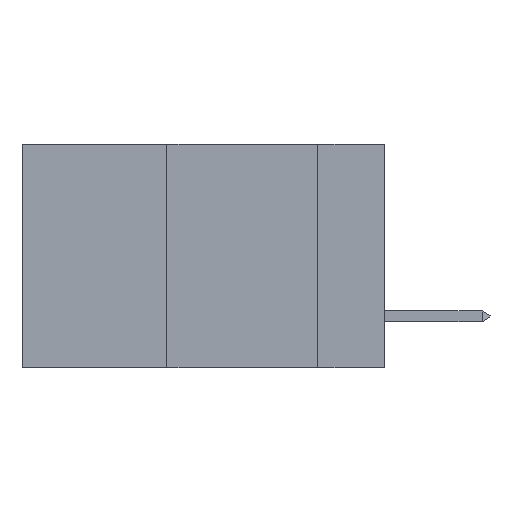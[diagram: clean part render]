
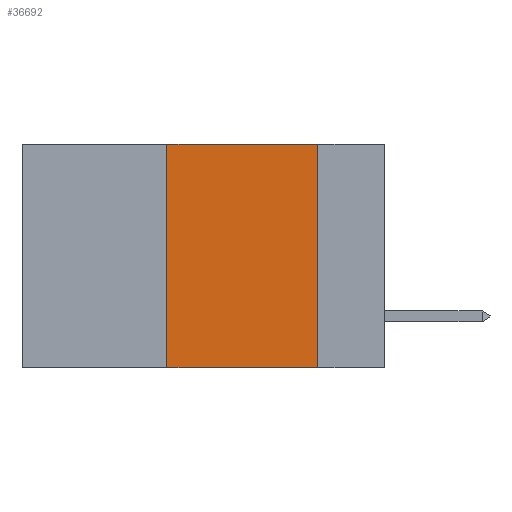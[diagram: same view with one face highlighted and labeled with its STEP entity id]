
A CAD part, left-side view. The second image highlights one B-rep face of the part: STEP entity #36692.
In plain terms, the highlighted planar face has unit normal (-1, 0, 0).
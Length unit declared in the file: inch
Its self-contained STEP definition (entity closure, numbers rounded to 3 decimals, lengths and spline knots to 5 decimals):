
#24 = LINE ( 'NONE', #11337, #18419 ) ;
#1571 = DIRECTION ( 'NONE',  ( 1., 0., 0. ) ) ;
#3225 = EDGE_CURVE ( 'NONE', #17568, #30742, #28594, .T. ) ;
#4828 = CARTESIAN_POINT ( 'NONE',  ( 0., 0.6, 0. ) ) ;
#4983 = LINE ( 'NONE', #13610, #28712 ) ;
#5018 = ORIENTED_EDGE ( 'NONE', *, *, #9924, .F. ) ;
#5063 = CARTESIAN_POINT ( 'NONE',  ( 0., 0.6, -0.37 ) ) ;
#5978 = VERTEX_POINT ( 'NONE', #36881 ) ;
#6490 = DIRECTION ( 'NONE',  ( 0., -1., 0. ) ) ;
#7766 = ORIENTED_EDGE ( 'NONE', *, *, #36840, .F. ) ;
#7857 = DIRECTION ( 'NONE',  ( 0., 0., 1. ) ) ;
#9007 = VECTOR ( 'NONE', #37203, 39.37008 ) ;
#9924 = EDGE_CURVE ( 'NONE', #17801, #5978, #35769, .T. ) ;
#10588 = FACE_OUTER_BOUND ( 'NONE', #22481, .T. ) ;
#11337 = CARTESIAN_POINT ( 'NONE',  ( 0., 0.11, 0. ) ) ;
#12231 = CARTESIAN_POINT ( 'NONE',  ( 0., 0.6, 0. ) ) ;
#13250 = DIRECTION ( 'NONE',  ( 0., 0., -1. ) ) ;
#13610 = CARTESIAN_POINT ( 'NONE',  ( 0., 0.36, 0. ) ) ;
#17288 = DIRECTION ( 'NONE',  ( 0., 0., -1. ) ) ;
#17568 = VERTEX_POINT ( 'NONE', #35295 ) ;
#17801 = VERTEX_POINT ( 'NONE', #18643 ) ;
#18419 = VECTOR ( 'NONE', #17288, 39.37008 ) ;
#18643 = CARTESIAN_POINT ( 'NONE',  ( 0., 0.36, 0. ) ) ;
#19626 = VECTOR ( 'NONE', #6490, 39.37008 ) ;
#22101 = CARTESIAN_POINT ( 'NONE',  ( 0., 0.11, -0.37 ) ) ;
#22481 = EDGE_LOOP ( 'NONE', ( #7766, #5018, #29814, #22827 ) ) ;
#22827 = ORIENTED_EDGE ( 'NONE', *, *, #3225, .T. ) ;
#25119 = PLANE ( 'NONE',  #34912 ) ;
#25186 = EDGE_CURVE ( 'NONE', #17568, #17801, #4983, .T. ) ;
#28594 = LINE ( 'NONE', #5063, #9007 ) ;
#28712 = VECTOR ( 'NONE', #7857, 39.37008 ) ;
#29814 = ORIENTED_EDGE ( 'NONE', *, *, #25186, .F. ) ;
#30742 = VERTEX_POINT ( 'NONE', #22101 ) ;
#34912 = AXIS2_PLACEMENT_3D ( 'NONE', #4828, #1571, #13250 ) ;
#35295 = CARTESIAN_POINT ( 'NONE',  ( 0., 0.36, -0.37 ) ) ;
#35769 = LINE ( 'NONE', #12231, #19626 ) ;
#36692 = ADVANCED_FACE ( 'NONE', ( #10588 ), #25119, .F. ) ;
#36840 = EDGE_CURVE ( 'NONE', #5978, #30742, #24, .T. ) ;
#36881 = CARTESIAN_POINT ( 'NONE',  ( 0., 0.11, 0. ) ) ;
#37203 = DIRECTION ( 'NONE',  ( 0., -1., 0. ) ) ;
